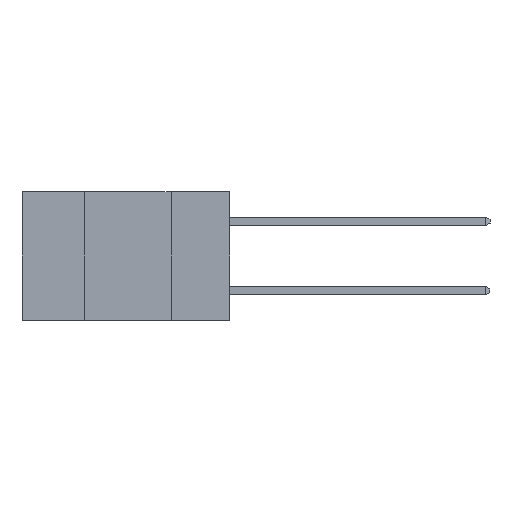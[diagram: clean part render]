
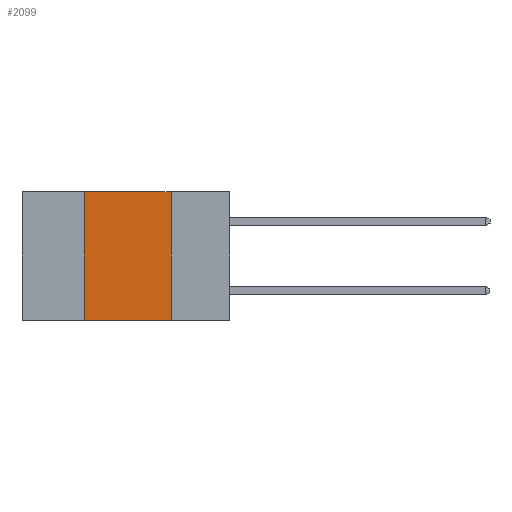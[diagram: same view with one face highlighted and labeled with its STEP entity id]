
A CAD part, left-side view. The second image highlights one B-rep face of the part: STEP entity #2099.
In plain terms, the highlighted planar face has unit normal (-1, 0, 0).
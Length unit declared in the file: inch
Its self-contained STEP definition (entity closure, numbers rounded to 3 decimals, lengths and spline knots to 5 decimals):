
#127 = LINE ( 'NONE', #9921, #11168 ) ;
#427 = ORIENTED_EDGE ( 'NONE', *, *, #5724, .F. ) ;
#809 = CARTESIAN_POINT ( 'NONE',  ( 0., 0.42, 0. ) ) ;
#961 = ORIENTED_EDGE ( 'NONE', *, *, #3681, .F. ) ;
#1672 = AXIS2_PLACEMENT_3D ( 'NONE', #17311, #16646, #6171 ) ;
#1929 = CARTESIAN_POINT ( 'NONE',  ( 0., 0.17, 0. ) ) ;
#2099 = ADVANCED_FACE ( 'NONE', ( #8229 ), #15385, .F. ) ;
#2754 = LINE ( 'NONE', #11348, #13327 ) ;
#3681 = EDGE_CURVE ( 'NONE', #12835, #16313, #12055, .T. ) ;
#4740 = CARTESIAN_POINT ( 'NONE',  ( 0., 0.42, -0.37 ) ) ;
#4854 = VECTOR ( 'NONE', #9474, 39.37008 ) ;
#5649 = CARTESIAN_POINT ( 'NONE',  ( 0., 0.17, 0. ) ) ;
#5724 = EDGE_CURVE ( 'NONE', #11834, #11318, #14559, .T. ) ;
#5862 = EDGE_LOOP ( 'NONE', ( #961, #16349, #427, #10323 ) ) ;
#6171 = DIRECTION ( 'NONE',  ( 0., 0., -1. ) ) ;
#6614 = EDGE_CURVE ( 'NONE', #11318, #12835, #127, .T. ) ;
#8229 = FACE_OUTER_BOUND ( 'NONE', #5862, .T. ) ;
#9474 = DIRECTION ( 'NONE',  ( 0., 0., -1. ) ) ;
#9921 = CARTESIAN_POINT ( 'NONE',  ( 0., 0.6, 0. ) ) ;
#10323 = ORIENTED_EDGE ( 'NONE', *, *, #14145, .T. ) ;
#11168 = VECTOR ( 'NONE', #11813, 39.37008 ) ;
#11318 = VERTEX_POINT ( 'NONE', #809 ) ;
#11348 = CARTESIAN_POINT ( 'NONE',  ( 0., 0.6, -0.37 ) ) ;
#11813 = DIRECTION ( 'NONE',  ( 0., -1., 0. ) ) ;
#11834 = VERTEX_POINT ( 'NONE', #4740 ) ;
#12055 = LINE ( 'NONE', #1929, #4854 ) ;
#12611 = CARTESIAN_POINT ( 'NONE',  ( 0., 0.17, -0.37 ) ) ;
#12835 = VERTEX_POINT ( 'NONE', #5649 ) ;
#13327 = VECTOR ( 'NONE', #15622, 39.37008 ) ;
#14106 = VECTOR ( 'NONE', #14960, 39.37008 ) ;
#14145 = EDGE_CURVE ( 'NONE', #11834, #16313, #2754, .T. ) ;
#14559 = LINE ( 'NONE', #14748, #14106 ) ;
#14748 = CARTESIAN_POINT ( 'NONE',  ( 0., 0.42, 0. ) ) ;
#14960 = DIRECTION ( 'NONE',  ( 0., 0., 1. ) ) ;
#15385 = PLANE ( 'NONE',  #1672 ) ;
#15622 = DIRECTION ( 'NONE',  ( 0., -1., 0. ) ) ;
#16313 = VERTEX_POINT ( 'NONE', #12611 ) ;
#16349 = ORIENTED_EDGE ( 'NONE', *, *, #6614, .F. ) ;
#16646 = DIRECTION ( 'NONE',  ( 1., 0., 0. ) ) ;
#17311 = CARTESIAN_POINT ( 'NONE',  ( 0., 0.6, 0. ) ) ;
